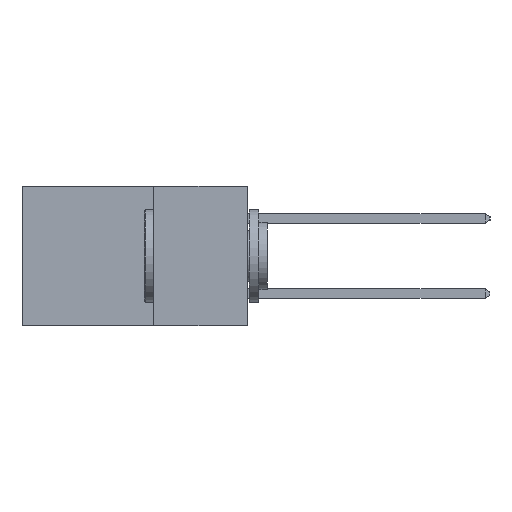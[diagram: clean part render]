
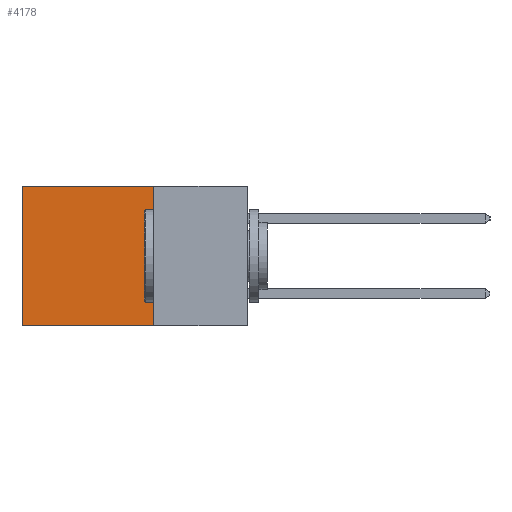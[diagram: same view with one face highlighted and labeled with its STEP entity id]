
A CAD part, left-side view. The second image highlights one B-rep face of the part: STEP entity #4178.
In plain terms, the highlighted planar face has unit normal (-1, 0, 0).
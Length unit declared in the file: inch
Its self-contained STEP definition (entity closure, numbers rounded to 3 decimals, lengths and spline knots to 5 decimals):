
#1454 = EDGE_CURVE ( 'NONE', #9295, #25185, #10661, .T. ) ;
#1496 = CARTESIAN_POINT ( 'NONE',  ( 0.2615, 0.25, 0. ) ) ;
#1559 = AXIS2_PLACEMENT_3D ( 'NONE', #11810, #15990, #3318 ) ;
#2270 = ORIENTED_EDGE ( 'NONE', *, *, #21854, .T. ) ;
#3318 = DIRECTION ( 'NONE',  ( 0., 0., -1. ) ) ;
#3699 = DIRECTION ( 'NONE',  ( 0., 1., 0. ) ) ;
#3801 = VECTOR ( 'NONE', #4537, 39.37008 ) ;
#4178 = ADVANCED_FACE ( 'NONE', ( #27010 ), #24205, .F. ) ;
#4195 = VERTEX_POINT ( 'NONE', #11889 ) ;
#4537 = DIRECTION ( 'NONE',  ( 0., 0., -1. ) ) ;
#5160 = LINE ( 'NONE', #8793, #3801 ) ;
#5169 = ORIENTED_EDGE ( 'NONE', *, *, #16931, .F. ) ;
#5754 = VECTOR ( 'NONE', #3699, 39.37008 ) ;
#6918 = CARTESIAN_POINT ( 'NONE',  ( 0.2615, 0.25, -0.37 ) ) ;
#7862 = CARTESIAN_POINT ( 'NONE',  ( 0.2615, 0.25, 0. ) ) ;
#8793 = CARTESIAN_POINT ( 'NONE',  ( 0.2615, 0.6, -0.37 ) ) ;
#8978 = CARTESIAN_POINT ( 'NONE',  ( 0.2615, 0.25, -0.37 ) ) ;
#9295 = VERTEX_POINT ( 'NONE', #7862 ) ;
#9832 = DIRECTION ( 'NONE',  ( 0., 0., -1. ) ) ;
#10193 = CARTESIAN_POINT ( 'NONE',  ( 0.2615, 0.25, -0.37 ) ) ;
#10661 = LINE ( 'NONE', #10193, #21090 ) ;
#11101 = DIRECTION ( 'NONE',  ( 0., 1., 0. ) ) ;
#11810 = CARTESIAN_POINT ( 'NONE',  ( 0.2615, 0.25, -0.37 ) ) ;
#11889 = CARTESIAN_POINT ( 'NONE',  ( 0.2615, 0.6, -0.37 ) ) ;
#14709 = VERTEX_POINT ( 'NONE', #18593 ) ;
#15990 = DIRECTION ( 'NONE',  ( 1., 0., 0. ) ) ;
#16266 = ORIENTED_EDGE ( 'NONE', *, *, #1454, .F. ) ;
#16931 = EDGE_CURVE ( 'NONE', #25185, #4195, #20560, .T. ) ;
#16960 = LINE ( 'NONE', #1496, #5754 ) ;
#18593 = CARTESIAN_POINT ( 'NONE',  ( 0.2615, 0.6, 0. ) ) ;
#19419 = EDGE_LOOP ( 'NONE', ( #24418, #5169, #16266, #2270 ) ) ;
#20560 = LINE ( 'NONE', #8978, #25313 ) ;
#21090 = VECTOR ( 'NONE', #9832, 39.37008 ) ;
#21854 = EDGE_CURVE ( 'NONE', #9295, #14709, #16960, .T. ) ;
#24205 = PLANE ( 'NONE',  #1559 ) ;
#24418 = ORIENTED_EDGE ( 'NONE', *, *, #26758, .T. ) ;
#25185 = VERTEX_POINT ( 'NONE', #6918 ) ;
#25313 = VECTOR ( 'NONE', #11101, 39.37008 ) ;
#26758 = EDGE_CURVE ( 'NONE', #14709, #4195, #5160, .T. ) ;
#27010 = FACE_OUTER_BOUND ( 'NONE', #19419, .T. ) ;
